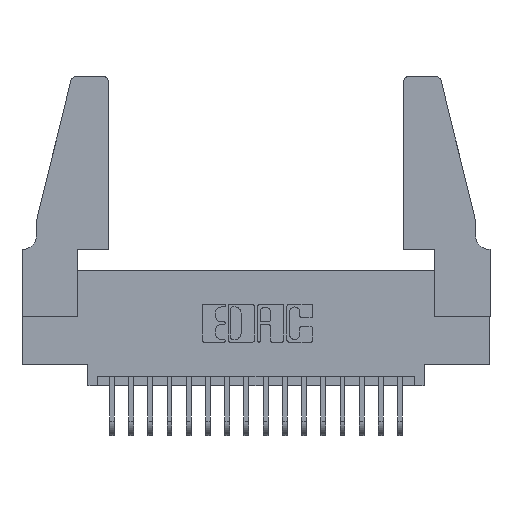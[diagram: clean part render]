
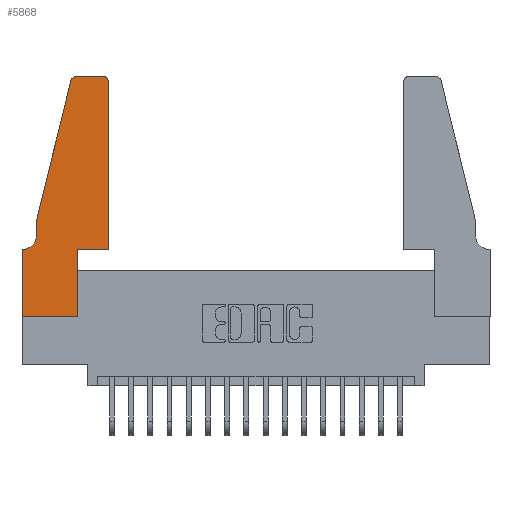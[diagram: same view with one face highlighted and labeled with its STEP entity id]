
A CAD part, top view. The second image highlights one B-rep face of the part: STEP entity #5868.
In plain terms, the highlighted planar face has unit normal (0, 0, 1).
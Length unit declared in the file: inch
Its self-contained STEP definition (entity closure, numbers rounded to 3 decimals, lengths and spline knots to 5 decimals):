
#57 = AXIS2_PLACEMENT_3D ( 'NONE', #13744, #4575, #15282 ) ;
#731 = ORIENTED_EDGE ( 'NONE', *, *, #4616, .T. ) ;
#736 = DIRECTION ( 'NONE',  ( 1., 0., 0. ) ) ;
#784 = DIRECTION ( 'NONE',  ( 0., -1., 0. ) ) ;
#1046 = VECTOR ( 'NONE', #18423, 39.37008 ) ;
#1076 = VERTEX_POINT ( 'NONE', #6065 ) ;
#1156 = CARTESIAN_POINT ( 'NONE',  ( 0., 0.35, 0.37 ) ) ;
#1190 = CARTESIAN_POINT ( 'NONE',  ( 0.4505, 1.22, 0.37 ) ) ;
#1250 = DIRECTION ( 'NONE',  ( -1., 0., 0. ) ) ;
#1588 = DIRECTION ( 'NONE',  ( 0., 1., 0. ) ) ;
#1789 = VERTEX_POINT ( 'NONE', #8786 ) ;
#1977 = ORIENTED_EDGE ( 'NONE', *, *, #14232, .T. ) ;
#2054 = EDGE_CURVE ( 'NONE', #4304, #1076, #9562, .T. ) ;
#2063 = ORIENTED_EDGE ( 'NONE', *, *, #8483, .T. ) ;
#2081 = CIRCLE ( 'NONE', #3431, 0.03 ) ;
#2150 = DIRECTION ( 'NONE',  ( 0., 0., 1. ) ) ;
#2569 = ORIENTED_EDGE ( 'NONE', *, *, #5524, .T. ) ;
#3136 = VECTOR ( 'NONE', #784, 39.37008 ) ;
#3431 = AXIS2_PLACEMENT_3D ( 'NONE', #19241, #10108, #736 ) ;
#3433 = CARTESIAN_POINT ( 'NONE',  ( 0.0055, 0.35, 0.37 ) ) ;
#3536 = CIRCLE ( 'NONE', #14250, 0.07 ) ;
#3834 = LINE ( 'NONE', #19972, #8932 ) ;
#3838 = LINE ( 'NONE', #6552, #19662 ) ;
#4304 = VERTEX_POINT ( 'NONE', #9437 ) ;
#4575 = DIRECTION ( 'NONE',  ( 0., 0., 1. ) ) ;
#4599 = DIRECTION ( 'NONE',  ( 0., 1., 0. ) ) ;
#4616 = EDGE_CURVE ( 'NONE', #5465, #6027, #19463, .T. ) ;
#5099 = LINE ( 'NONE', #6168, #12728 ) ;
#5126 = AXIS2_PLACEMENT_3D ( 'NONE', #11399, #2150, #12935 ) ;
#5465 = VERTEX_POINT ( 'NONE', #7440 ) ;
#5524 = EDGE_CURVE ( 'NONE', #13231, #14136, #18954, .T. ) ;
#5688 = VERTEX_POINT ( 'NONE', #9520 ) ;
#5723 = ORIENTED_EDGE ( 'NONE', *, *, #11404, .T. ) ;
#5764 = ORIENTED_EDGE ( 'NONE', *, *, #12617, .T. ) ;
#5868 = ADVANCED_FACE ( 'NONE', ( #13101 ), #19047, .T. ) ;
#6027 = VERTEX_POINT ( 'NONE', #17885 ) ;
#6065 = CARTESIAN_POINT ( 'NONE',  ( 0.2865, 0.35, 0.37 ) ) ;
#6133 = CARTESIAN_POINT ( 'NONE',  ( 0.0055, 0.42, 0.37 ) ) ;
#6168 = CARTESIAN_POINT ( 'NONE',  ( 0.4505, 0.35, 0.37 ) ) ;
#6332 = VECTOR ( 'NONE', #14612, 39.37008 ) ;
#6552 = CARTESIAN_POINT ( 'NONE',  ( 0.2605, 1.25, 0.37 ) ) ;
#6767 = VECTOR ( 'NONE', #1250, 39.37008 ) ;
#7062 = CARTESIAN_POINT ( 'NONE',  ( 0., 0., 0.37 ) ) ;
#7310 = EDGE_LOOP ( 'NONE', ( #11805, #19015, #2063, #731, #1977, #2569, #5764, #7428, #10936, #5723, #8718, #11014 ) ) ;
#7428 = ORIENTED_EDGE ( 'NONE', *, *, #14660, .T. ) ;
#7440 = CARTESIAN_POINT ( 'NONE',  ( 0.0755, 0.5, 0.37 ) ) ;
#7673 = DIRECTION ( 'NONE',  ( -1., 0., 0. ) ) ;
#7750 = CARTESIAN_POINT ( 'NONE',  ( 0.4205, 1.25, 0.37 ) ) ;
#8133 = VECTOR ( 'NONE', #16172, 39.37008 ) ;
#8483 = EDGE_CURVE ( 'NONE', #9670, #5465, #18030, .T. ) ;
#8718 = ORIENTED_EDGE ( 'NONE', *, *, #9461, .T. ) ;
#8786 = CARTESIAN_POINT ( 'NONE',  ( 0.284, 1.25, 0.37 ) ) ;
#8932 = VECTOR ( 'NONE', #9328, 39.37008 ) ;
#9328 = DIRECTION ( 'NONE',  ( 0., -1., 0. ) ) ;
#9383 = CARTESIAN_POINT ( 'NONE',  ( 0.2865, 0.35, 0.37 ) ) ;
#9437 = CARTESIAN_POINT ( 'NONE',  ( 0.2865, 0., 0.37 ) ) ;
#9461 = EDGE_CURVE ( 'NONE', #16797, #12466, #5099, .T. ) ;
#9520 = CARTESIAN_POINT ( 'NONE',  ( 0., 0., 0.37 ) ) ;
#9562 = LINE ( 'NONE', #9383, #12601 ) ;
#9670 = VERTEX_POINT ( 'NONE', #9719 ) ;
#9719 = CARTESIAN_POINT ( 'NONE',  ( 0.25487, 1.22718, 0.37 ) ) ;
#10108 = DIRECTION ( 'NONE',  ( 0., 0., 1. ) ) ;
#10188 = EDGE_CURVE ( 'NONE', #11417, #1789, #3838, .T. ) ;
#10559 = CARTESIAN_POINT ( 'NONE',  ( 0.0755, 0.35, 0.37 ) ) ;
#10936 = ORIENTED_EDGE ( 'NONE', *, *, #2054, .T. ) ;
#11014 = ORIENTED_EDGE ( 'NONE', *, *, #12963, .T. ) ;
#11129 = DIRECTION ( 'NONE',  ( -1., 0., 0. ) ) ;
#11399 = CARTESIAN_POINT ( 'NONE',  ( 0., 0.35, 0.37 ) ) ;
#11404 = EDGE_CURVE ( 'NONE', #1076, #16797, #13878, .T. ) ;
#11417 = VERTEX_POINT ( 'NONE', #7750 ) ;
#11805 = ORIENTED_EDGE ( 'NONE', *, *, #10188, .T. ) ;
#12466 = VERTEX_POINT ( 'NONE', #1190 ) ;
#12601 = VECTOR ( 'NONE', #1588, 39.37008 ) ;
#12617 = EDGE_CURVE ( 'NONE', #14136, #5688, #3834, .T. ) ;
#12728 = VECTOR ( 'NONE', #4599, 39.37008 ) ;
#12935 = DIRECTION ( 'NONE',  ( 1., 0., 0. ) ) ;
#12963 = EDGE_CURVE ( 'NONE', #12466, #11417, #2081, .T. ) ;
#13052 = CARTESIAN_POINT ( 'NONE',  ( 0.0755, 0.5, 0.37 ) ) ;
#13101 = FACE_OUTER_BOUND ( 'NONE', #7310, .T. ) ;
#13144 = CIRCLE ( 'NONE', #57, 0.03 ) ;
#13231 = VERTEX_POINT ( 'NONE', #3433 ) ;
#13697 = EDGE_CURVE ( 'NONE', #1789, #9670, #13144, .T. ) ;
#13744 = CARTESIAN_POINT ( 'NONE',  ( 0.284, 1.22, 0.37 ) ) ;
#13803 = CARTESIAN_POINT ( 'NONE',  ( 0.4505, 0.35, 0.37 ) ) ;
#13878 = LINE ( 'NONE', #13803, #1046 ) ;
#14136 = VERTEX_POINT ( 'NONE', #1156 ) ;
#14232 = EDGE_CURVE ( 'NONE', #6027, #13231, #3536, .T. ) ;
#14250 = AXIS2_PLACEMENT_3D ( 'NONE', #6133, #16794, #7673 ) ;
#14612 = DIRECTION ( 'NONE',  ( -0.239, -0.971, 0. ) ) ;
#14660 = EDGE_CURVE ( 'NONE', #5688, #4304, #16209, .T. ) ;
#15282 = DIRECTION ( 'NONE',  ( 1., 0., 0. ) ) ;
#16172 = DIRECTION ( 'NONE',  ( 1., 0., 0. ) ) ;
#16209 = LINE ( 'NONE', #7062, #8133 ) ;
#16410 = CARTESIAN_POINT ( 'NONE',  ( 0.4505, 0.35, 0.37 ) ) ;
#16794 = DIRECTION ( 'NONE',  ( 0., 0., -1. ) ) ;
#16797 = VERTEX_POINT ( 'NONE', #16410 ) ;
#17738 = CARTESIAN_POINT ( 'NONE',  ( 0.0755, 0.5, 0.37 ) ) ;
#17885 = CARTESIAN_POINT ( 'NONE',  ( 0.0755, 0.42, 0.37 ) ) ;
#18030 = LINE ( 'NONE', #13052, #6332 ) ;
#18423 = DIRECTION ( 'NONE',  ( 1., 0., 0. ) ) ;
#18954 = LINE ( 'NONE', #10559, #6767 ) ;
#19015 = ORIENTED_EDGE ( 'NONE', *, *, #13697, .T. ) ;
#19047 = PLANE ( 'NONE',  #5126 ) ;
#19241 = CARTESIAN_POINT ( 'NONE',  ( 0.4205, 1.22, 0.37 ) ) ;
#19463 = LINE ( 'NONE', #17738, #3136 ) ;
#19662 = VECTOR ( 'NONE', #11129, 39.37008 ) ;
#19972 = CARTESIAN_POINT ( 'NONE',  ( 0., 0., 0.37 ) ) ;
